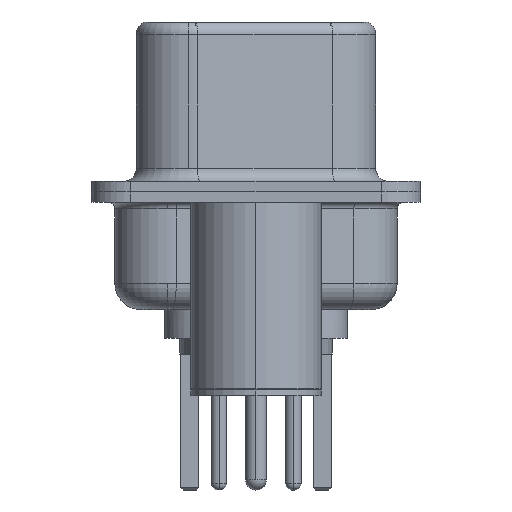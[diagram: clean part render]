
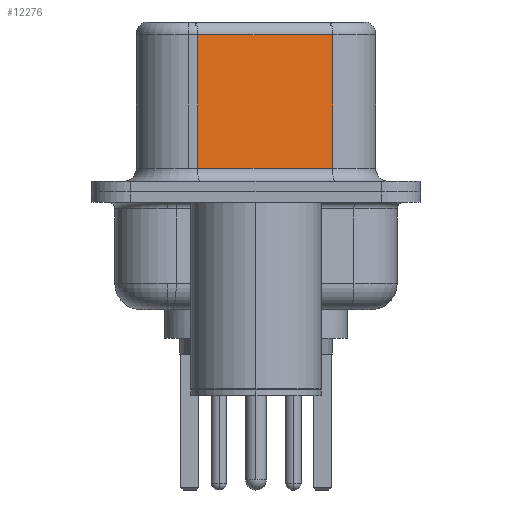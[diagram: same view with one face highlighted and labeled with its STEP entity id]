
A CAD part, left-side view. The second image highlights one B-rep face of the part: STEP entity #12276.
In plain terms, the highlighted planar face has unit normal (-0.985, -0.174, 0).
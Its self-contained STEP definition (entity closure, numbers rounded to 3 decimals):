
#172 = LINE ( 'NONE', #5166, #20765 ) ;
#428 = PLANE ( 'NONE',  #18377 ) ;
#1084 = CARTESIAN_POINT ( 'NONE',  ( 3.67, 2.233, 0.9 ) ) ;
#2723 = DIRECTION ( 'NONE',  ( 0., 0., -1. ) ) ;
#5151 = ORIENTED_EDGE ( 'NONE', *, *, #21774, .T. ) ;
#5166 = CARTESIAN_POINT ( 'NONE',  ( 4.58, -2.927, 6.52 ) ) ;
#5385 = VERTEX_POINT ( 'NONE', #27065 ) ;
#6065 = LINE ( 'NONE', #20737, #22865 ) ;
#6658 = VECTOR ( 'NONE', #2723, 1000. ) ;
#7308 = CARTESIAN_POINT ( 'NONE',  ( 3.67, 2.233, 6.52 ) ) ;
#8918 = VERTEX_POINT ( 'NONE', #23928 ) ;
#8978 = LINE ( 'NONE', #10434, #19988 ) ;
#9234 = DIRECTION ( 'NONE',  ( 0.985, 0.174, 0. ) ) ;
#9255 = EDGE_CURVE ( 'NONE', #5385, #10019, #172, .T. ) ;
#10019 = VERTEX_POINT ( 'NONE', #10864 ) ;
#10170 = EDGE_LOOP ( 'NONE', ( #26867, #23659, #27355, #5151 ) ) ;
#10434 = CARTESIAN_POINT ( 'NONE',  ( 4.58, -2.927, 6.02 ) ) ;
#10864 = CARTESIAN_POINT ( 'NONE',  ( 4.58, -2.927, 0.9 ) ) ;
#11749 = LINE ( 'NONE', #7308, #6658 ) ;
#12091 = FACE_OUTER_BOUND ( 'NONE', #10170, .T. ) ;
#12276 = ADVANCED_FACE ( 'NONE', ( #12091 ), #428, .F. ) ;
#12431 = VERTEX_POINT ( 'NONE', #1084 ) ;
#13480 = EDGE_CURVE ( 'NONE', #8918, #12431, #11749, .T. ) ;
#17984 = CARTESIAN_POINT ( 'NONE',  ( 4.58, -2.927, 6.52 ) ) ;
#18377 = AXIS2_PLACEMENT_3D ( 'NONE', #17984, #9234, #24561 ) ;
#19988 = VECTOR ( 'NONE', #25755, 1000. ) ;
#20737 = CARTESIAN_POINT ( 'NONE',  ( 4.58, -2.927, 0.9 ) ) ;
#20765 = VECTOR ( 'NONE', #21872, 1000. ) ;
#21774 = EDGE_CURVE ( 'NONE', #12431, #10019, #6065, .T. ) ;
#21872 = DIRECTION ( 'NONE',  ( 0., 0., -1. ) ) ;
#22865 = VECTOR ( 'NONE', #22919, 1000. ) ;
#22919 = DIRECTION ( 'NONE',  ( 0.174, -0.985, 0. ) ) ;
#23659 = ORIENTED_EDGE ( 'NONE', *, *, #25345, .T. ) ;
#23928 = CARTESIAN_POINT ( 'NONE',  ( 3.67, 2.233, 6.02 ) ) ;
#24561 = DIRECTION ( 'NONE',  ( -0.174, 0.985, 0. ) ) ;
#25345 = EDGE_CURVE ( 'NONE', #5385, #8918, #8978, .T. ) ;
#25755 = DIRECTION ( 'NONE',  ( -0.174, 0.985, 0. ) ) ;
#26867 = ORIENTED_EDGE ( 'NONE', *, *, #9255, .F. ) ;
#27065 = CARTESIAN_POINT ( 'NONE',  ( 4.58, -2.927, 6.02 ) ) ;
#27355 = ORIENTED_EDGE ( 'NONE', *, *, #13480, .T. ) ;
